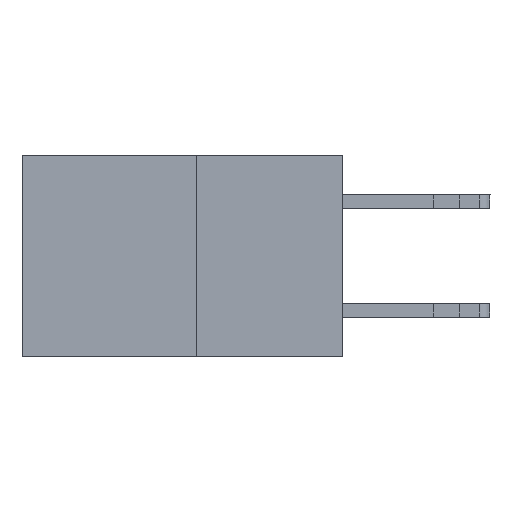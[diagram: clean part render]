
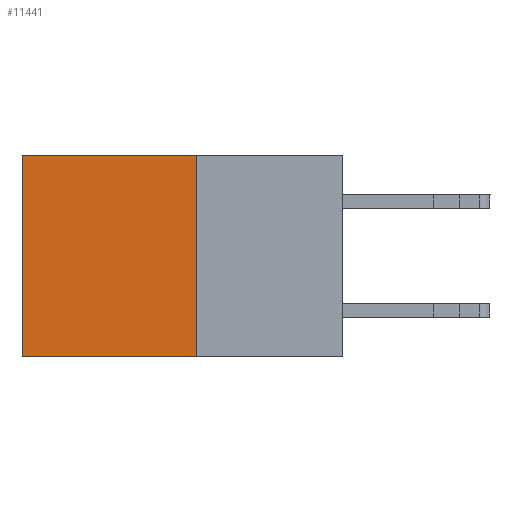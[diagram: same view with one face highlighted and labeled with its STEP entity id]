
A CAD part, left-side view. The second image highlights one B-rep face of the part: STEP entity #11441.
In plain terms, the highlighted planar face has unit normal (-1, 0, 0).
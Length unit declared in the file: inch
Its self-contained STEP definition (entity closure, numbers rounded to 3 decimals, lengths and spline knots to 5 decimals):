
#50 = CARTESIAN_POINT ( 'NONE',  ( 0.277, 0.27, -0.37 ) ) ;
#79 = DIRECTION ( 'NONE',  ( 0., 1., 0. ) ) ;
#94 = CARTESIAN_POINT ( 'NONE',  ( 0.277, 0.59, 0. ) ) ;
#97 = LINE ( 'NONE', #9593, #10633 ) ;
#922 = CARTESIAN_POINT ( 'NONE',  ( 0.277, 0.27, -0.37 ) ) ;
#1313 = DIRECTION ( 'NONE',  ( 0., 0., -1. ) ) ;
#1339 = DIRECTION ( 'NONE',  ( 0., 0., -1. ) ) ;
#2163 = ORIENTED_EDGE ( 'NONE', *, *, #5928, .F. ) ;
#2469 = FACE_OUTER_BOUND ( 'NONE', #12993, .T. ) ;
#3058 = VECTOR ( 'NONE', #79, 39.37008 ) ;
#3420 = DIRECTION ( 'NONE',  ( 0., 0., -1. ) ) ;
#4657 = DIRECTION ( 'NONE',  ( 1., 0., 0. ) ) ;
#5514 = VECTOR ( 'NONE', #11603, 39.37008 ) ;
#5563 = ORIENTED_EDGE ( 'NONE', *, *, #6367, .T. ) ;
#5928 = EDGE_CURVE ( 'NONE', #10253, #10804, #9824, .T. ) ;
#5948 = PLANE ( 'NONE',  #9910 ) ;
#6367 = EDGE_CURVE ( 'NONE', #15548, #10804, #97, .T. ) ;
#7057 = EDGE_CURVE ( 'NONE', #9518, #15548, #13121, .T. ) ;
#8349 = CARTESIAN_POINT ( 'NONE',  ( 0.277, 0.27, -0.37 ) ) ;
#9444 = CARTESIAN_POINT ( 'NONE',  ( 0.277, 0.27, 0. ) ) ;
#9518 = VERTEX_POINT ( 'NONE', #9444 ) ;
#9593 = CARTESIAN_POINT ( 'NONE',  ( 0.277, 0.59, -0.37 ) ) ;
#9824 = LINE ( 'NONE', #13724, #3058 ) ;
#9910 = AXIS2_PLACEMENT_3D ( 'NONE', #922, #4657, #3420 ) ;
#10253 = VERTEX_POINT ( 'NONE', #8349 ) ;
#10454 = CARTESIAN_POINT ( 'NONE',  ( 0.277, 0.27, 0. ) ) ;
#10633 = VECTOR ( 'NONE', #1313, 39.37008 ) ;
#10804 = VERTEX_POINT ( 'NONE', #15581 ) ;
#11159 = LINE ( 'NONE', #50, #13600 ) ;
#11266 = ORIENTED_EDGE ( 'NONE', *, *, #7057, .T. ) ;
#11441 = ADVANCED_FACE ( 'NONE', ( #2469 ), #5948, .F. ) ;
#11603 = DIRECTION ( 'NONE',  ( 0., 1., 0. ) ) ;
#11609 = ORIENTED_EDGE ( 'NONE', *, *, #13355, .F. ) ;
#12993 = EDGE_LOOP ( 'NONE', ( #5563, #2163, #11609, #11266 ) ) ;
#13121 = LINE ( 'NONE', #10454, #5514 ) ;
#13355 = EDGE_CURVE ( 'NONE', #9518, #10253, #11159, .T. ) ;
#13600 = VECTOR ( 'NONE', #1339, 39.37008 ) ;
#13724 = CARTESIAN_POINT ( 'NONE',  ( 0.277, 0.27, -0.37 ) ) ;
#15548 = VERTEX_POINT ( 'NONE', #94 ) ;
#15581 = CARTESIAN_POINT ( 'NONE',  ( 0.277, 0.59, -0.37 ) ) ;
